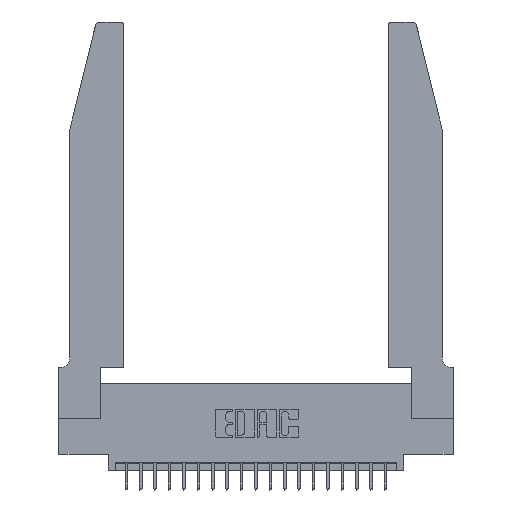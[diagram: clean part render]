
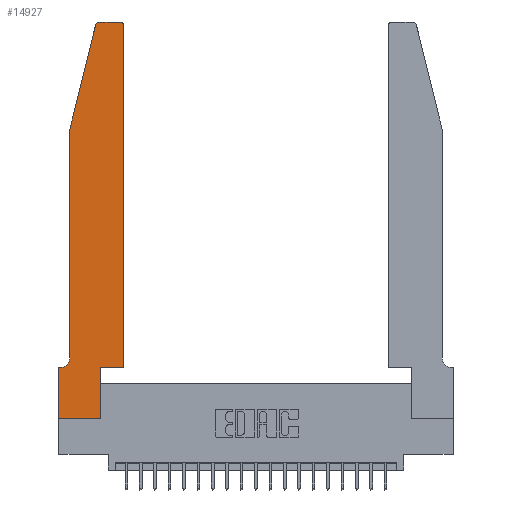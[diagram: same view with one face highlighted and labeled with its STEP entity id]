
A CAD part, top view. The second image highlights one B-rep face of the part: STEP entity #14927.
In plain terms, the highlighted planar face has unit normal (0, 0, 1).
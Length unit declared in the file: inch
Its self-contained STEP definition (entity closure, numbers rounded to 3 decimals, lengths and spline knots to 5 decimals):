
#335 = CARTESIAN_POINT ( 'NONE',  ( 0.0755, 2., 0.37 ) ) ;
#392 = CARTESIAN_POINT ( 'NONE',  ( 0.284, 2.75, 0.37 ) ) ;
#562 = LINE ( 'NONE', #335, #5155 ) ;
#1439 = CIRCLE ( 'NONE', #17054, 0.03 ) ;
#1595 = DIRECTION ( 'NONE',  ( 0., 1., 0. ) ) ;
#1664 = DIRECTION ( 'NONE',  ( 0., 0., -1. ) ) ;
#1697 = VECTOR ( 'NONE', #3751, 39.37008 ) ;
#1776 = ORIENTED_EDGE ( 'NONE', *, *, #4009, .T. ) ;
#1830 = ORIENTED_EDGE ( 'NONE', *, *, #22244, .T. ) ;
#2185 = VECTOR ( 'NONE', #8584, 39.37008 ) ;
#2213 = ORIENTED_EDGE ( 'NONE', *, *, #21782, .T. ) ;
#2255 = DIRECTION ( 'NONE',  ( 1., 0., 0. ) ) ;
#2305 = CARTESIAN_POINT ( 'NONE',  ( 0.2865, 0.35, 0.37 ) ) ;
#2401 = CARTESIAN_POINT ( 'NONE',  ( 0.0755, 0.42, 0.37 ) ) ;
#2495 = VERTEX_POINT ( 'NONE', #16827 ) ;
#2776 = CARTESIAN_POINT ( 'NONE',  ( 0., 0., 0.37 ) ) ;
#2904 = EDGE_CURVE ( 'NONE', #4627, #14801, #6862, .T. ) ;
#3347 = CARTESIAN_POINT ( 'NONE',  ( 0.4505, 0.35, 0.37 ) ) ;
#3548 = ORIENTED_EDGE ( 'NONE', *, *, #22206, .T. ) ;
#3580 = ORIENTED_EDGE ( 'NONE', *, *, #15104, .T. ) ;
#3751 = DIRECTION ( 'NONE',  ( 1., 0., 0. ) ) ;
#4009 = EDGE_CURVE ( 'NONE', #2495, #11284, #10470, .T. ) ;
#4227 = DIRECTION ( 'NONE',  ( -1., 0., 0. ) ) ;
#4294 = VERTEX_POINT ( 'NONE', #14283 ) ;
#4627 = VERTEX_POINT ( 'NONE', #15027 ) ;
#4697 = CARTESIAN_POINT ( 'NONE',  ( 0., 0., 0.37 ) ) ;
#4769 = CARTESIAN_POINT ( 'NONE',  ( 0.25487, 2.72718, 0.37 ) ) ;
#4951 = CARTESIAN_POINT ( 'NONE',  ( 0.2865, 0., 0.37 ) ) ;
#5155 = VECTOR ( 'NONE', #7452, 39.37008 ) ;
#5180 = CARTESIAN_POINT ( 'NONE',  ( 0.4505, 2.72, 0.37 ) ) ;
#5243 = CARTESIAN_POINT ( 'NONE',  ( 0.2605, 2.75, 0.37 ) ) ;
#5576 = CARTESIAN_POINT ( 'NONE',  ( 0.4205, 2.75, 0.37 ) ) ;
#5859 = VERTEX_POINT ( 'NONE', #5576 ) ;
#6683 = ORIENTED_EDGE ( 'NONE', *, *, #21516, .T. ) ;
#6862 = LINE ( 'NONE', #17801, #13105 ) ;
#7021 = CIRCLE ( 'NONE', #20365, 0.03 ) ;
#7066 = EDGE_CURVE ( 'NONE', #22555, #4627, #562, .T. ) ;
#7203 = VERTEX_POINT ( 'NONE', #2776 ) ;
#7274 = CARTESIAN_POINT ( 'NONE',  ( 0.4205, 2.72, 0.37 ) ) ;
#7452 = DIRECTION ( 'NONE',  ( -0.239, -0.971, 0. ) ) ;
#7724 = VERTEX_POINT ( 'NONE', #392 ) ;
#7884 = DIRECTION ( 'NONE',  ( 0., -1., 0. ) ) ;
#8342 = ORIENTED_EDGE ( 'NONE', *, *, #16003, .T. ) ;
#8490 = CARTESIAN_POINT ( 'NONE',  ( 0.4505, 0.35, 0.37 ) ) ;
#8584 = DIRECTION ( 'NONE',  ( 0., 1., 0. ) ) ;
#8839 = ORIENTED_EDGE ( 'NONE', *, *, #10578, .T. ) ;
#8852 = DIRECTION ( 'NONE',  ( 1., 0., 0. ) ) ;
#9744 = LINE ( 'NONE', #22140, #21194 ) ;
#10004 = LINE ( 'NONE', #13808, #2185 ) ;
#10032 = CARTESIAN_POINT ( 'NONE',  ( 0.0055, 0.35, 0.37 ) ) ;
#10061 = VERTEX_POINT ( 'NONE', #2305 ) ;
#10295 = PLANE ( 'NONE',  #21709 ) ;
#10398 = DIRECTION ( 'NONE',  ( -1., 0., 0. ) ) ;
#10470 = LINE ( 'NONE', #8490, #10547 ) ;
#10547 = VECTOR ( 'NONE', #1595, 39.37008 ) ;
#10578 = EDGE_CURVE ( 'NONE', #21075, #4294, #9744, .T. ) ;
#11004 = LINE ( 'NONE', #17963, #1697 ) ;
#11134 = CIRCLE ( 'NONE', #18175, 0.07 ) ;
#11284 = VERTEX_POINT ( 'NONE', #5180 ) ;
#11841 = VECTOR ( 'NONE', #10398, 39.37008 ) ;
#11898 = DIRECTION ( 'NONE',  ( 1., 0., 0. ) ) ;
#12078 = EDGE_LOOP ( 'NONE', ( #2213, #6683, #12541, #19908, #3548, #8839, #13785, #8342, #14437, #3580, #1776, #1830 ) ) ;
#12276 = LINE ( 'NONE', #4697, #15357 ) ;
#12386 = DIRECTION ( 'NONE',  ( 1., 0., 0. ) ) ;
#12541 = ORIENTED_EDGE ( 'NONE', *, *, #7066, .T. ) ;
#13105 = VECTOR ( 'NONE', #7884, 39.37008 ) ;
#13498 = EDGE_CURVE ( 'NONE', #4294, #7203, #12276, .T. ) ;
#13542 = CARTESIAN_POINT ( 'NONE',  ( 0., 0.35, 0.37 ) ) ;
#13785 = ORIENTED_EDGE ( 'NONE', *, *, #13498, .T. ) ;
#13808 = CARTESIAN_POINT ( 'NONE',  ( 0.2865, 0.35, 0.37 ) ) ;
#14283 = CARTESIAN_POINT ( 'NONE',  ( 0., 0.35, 0.37 ) ) ;
#14382 = DIRECTION ( 'NONE',  ( 0., 0., 1. ) ) ;
#14437 = ORIENTED_EDGE ( 'NONE', *, *, #21405, .T. ) ;
#14801 = VERTEX_POINT ( 'NONE', #2401 ) ;
#14834 = DIRECTION ( 'NONE',  ( 0., 0., 1. ) ) ;
#14927 = ADVANCED_FACE ( 'NONE', ( #17472 ), #10295, .T. ) ;
#15027 = CARTESIAN_POINT ( 'NONE',  ( 0.0755, 2., 0.37 ) ) ;
#15104 = EDGE_CURVE ( 'NONE', #10061, #2495, #21138, .T. ) ;
#15357 = VECTOR ( 'NONE', #18886, 39.37008 ) ;
#15734 = LINE ( 'NONE', #5243, #11841 ) ;
#15789 = VECTOR ( 'NONE', #8852, 39.37008 ) ;
#16003 = EDGE_CURVE ( 'NONE', #7203, #16753, #11004, .T. ) ;
#16753 = VERTEX_POINT ( 'NONE', #4951 ) ;
#16827 = CARTESIAN_POINT ( 'NONE',  ( 0.4505, 0.35, 0.37 ) ) ;
#17054 = AXIS2_PLACEMENT_3D ( 'NONE', #7274, #14382, #12386 ) ;
#17472 = FACE_OUTER_BOUND ( 'NONE', #12078, .T. ) ;
#17488 = DIRECTION ( 'NONE',  ( -1., 0., 0. ) ) ;
#17801 = CARTESIAN_POINT ( 'NONE',  ( 0.0755, 2., 0.37 ) ) ;
#17963 = CARTESIAN_POINT ( 'NONE',  ( 0., 0., 0.37 ) ) ;
#18175 = AXIS2_PLACEMENT_3D ( 'NONE', #20838, #1664, #17488 ) ;
#18311 = CARTESIAN_POINT ( 'NONE',  ( 0.284, 2.72, 0.37 ) ) ;
#18886 = DIRECTION ( 'NONE',  ( 0., -1., 0. ) ) ;
#19908 = ORIENTED_EDGE ( 'NONE', *, *, #2904, .T. ) ;
#20365 = AXIS2_PLACEMENT_3D ( 'NONE', #18311, #14834, #2255 ) ;
#20606 = DIRECTION ( 'NONE',  ( 0., 0., 1. ) ) ;
#20838 = CARTESIAN_POINT ( 'NONE',  ( 0.0055, 0.42, 0.37 ) ) ;
#21075 = VERTEX_POINT ( 'NONE', #10032 ) ;
#21138 = LINE ( 'NONE', #3347, #15789 ) ;
#21194 = VECTOR ( 'NONE', #4227, 39.37008 ) ;
#21405 = EDGE_CURVE ( 'NONE', #16753, #10061, #10004, .T. ) ;
#21516 = EDGE_CURVE ( 'NONE', #7724, #22555, #7021, .T. ) ;
#21709 = AXIS2_PLACEMENT_3D ( 'NONE', #13542, #20606, #11898 ) ;
#21782 = EDGE_CURVE ( 'NONE', #5859, #7724, #15734, .T. ) ;
#22140 = CARTESIAN_POINT ( 'NONE',  ( 0.0755, 0.35, 0.37 ) ) ;
#22206 = EDGE_CURVE ( 'NONE', #14801, #21075, #11134, .T. ) ;
#22244 = EDGE_CURVE ( 'NONE', #11284, #5859, #1439, .T. ) ;
#22555 = VERTEX_POINT ( 'NONE', #4769 ) ;
